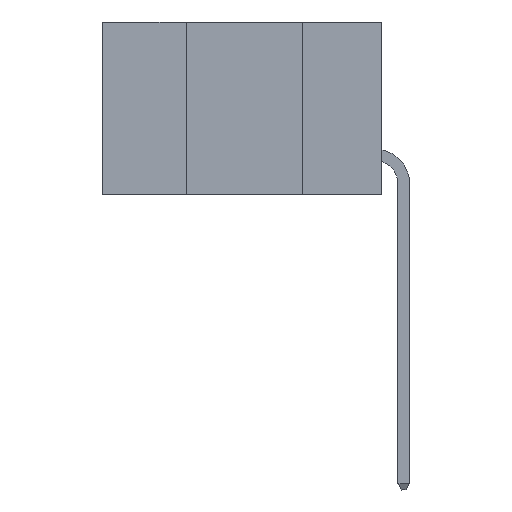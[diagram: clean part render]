
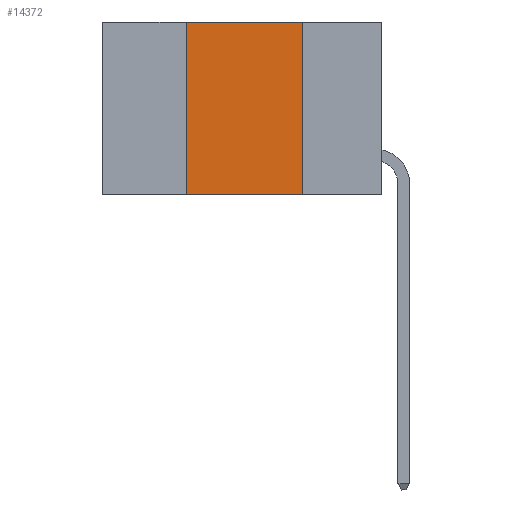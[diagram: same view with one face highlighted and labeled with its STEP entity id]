
A CAD part, left-side view. The second image highlights one B-rep face of the part: STEP entity #14372.
In plain terms, the highlighted planar face has unit normal (-1, 0, 0).
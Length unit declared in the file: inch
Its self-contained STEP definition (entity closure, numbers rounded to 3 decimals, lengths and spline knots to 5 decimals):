
#860 = VECTOR ( 'NONE', #23253, 39.37008 ) ;
#1283 = EDGE_CURVE ( 'NONE', #23550, #6151, #23429, .T. ) ;
#1407 = VERTEX_POINT ( 'NONE', #6427 ) ;
#1477 = LINE ( 'NONE', #4530, #860 ) ;
#1894 = ORIENTED_EDGE ( 'NONE', *, *, #17570, .F. ) ;
#3297 = CARTESIAN_POINT ( 'NONE',  ( 0., 0.42, 0. ) ) ;
#4530 = CARTESIAN_POINT ( 'NONE',  ( 0., 0.17, 0. ) ) ;
#4700 = VECTOR ( 'NONE', #9750, 39.37008 ) ;
#4800 = DIRECTION ( 'NONE',  ( 0., 0., -1. ) ) ;
#6151 = VERTEX_POINT ( 'NONE', #3297 ) ;
#6427 = CARTESIAN_POINT ( 'NONE',  ( 0., 0.17, -0.37 ) ) ;
#7527 = ORIENTED_EDGE ( 'NONE', *, *, #16145, .T. ) ;
#8339 = CARTESIAN_POINT ( 'NONE',  ( 0., 0.6, 0. ) ) ;
#9176 = CARTESIAN_POINT ( 'NONE',  ( 0., 0.17, 0. ) ) ;
#9750 = DIRECTION ( 'NONE',  ( 0., -1., 0. ) ) ;
#11408 = FACE_OUTER_BOUND ( 'NONE', #13101, .T. ) ;
#12465 = CARTESIAN_POINT ( 'NONE',  ( 0., 0.6, 0. ) ) ;
#12761 = AXIS2_PLACEMENT_3D ( 'NONE', #12465, #16162, #4800 ) ;
#13101 = EDGE_LOOP ( 'NONE', ( #18230, #1894, #14459, #7527 ) ) ;
#14244 = LINE ( 'NONE', #22668, #4700 ) ;
#14372 = ADVANCED_FACE ( 'NONE', ( #11408 ), #17868, .F. ) ;
#14459 = ORIENTED_EDGE ( 'NONE', *, *, #1283, .F. ) ;
#14661 = CARTESIAN_POINT ( 'NONE',  ( 0., 0.42, 0. ) ) ;
#15931 = VERTEX_POINT ( 'NONE', #9176 ) ;
#16145 = EDGE_CURVE ( 'NONE', #23550, #1407, #14244, .T. ) ;
#16162 = DIRECTION ( 'NONE',  ( 1., 0., 0. ) ) ;
#17570 = EDGE_CURVE ( 'NONE', #6151, #15931, #18715, .T. ) ;
#17604 = DIRECTION ( 'NONE',  ( 0., -1., 0. ) ) ;
#17868 = PLANE ( 'NONE',  #12761 ) ;
#18230 = ORIENTED_EDGE ( 'NONE', *, *, #23218, .F. ) ;
#18528 = VECTOR ( 'NONE', #22914, 39.37008 ) ;
#18637 = CARTESIAN_POINT ( 'NONE',  ( 0., 0.42, -0.37 ) ) ;
#18715 = LINE ( 'NONE', #8339, #19301 ) ;
#19301 = VECTOR ( 'NONE', #17604, 39.37008 ) ;
#22668 = CARTESIAN_POINT ( 'NONE',  ( 0., 0.6, -0.37 ) ) ;
#22914 = DIRECTION ( 'NONE',  ( 0., 0., 1. ) ) ;
#23218 = EDGE_CURVE ( 'NONE', #15931, #1407, #1477, .T. ) ;
#23253 = DIRECTION ( 'NONE',  ( 0., 0., -1. ) ) ;
#23429 = LINE ( 'NONE', #14661, #18528 ) ;
#23550 = VERTEX_POINT ( 'NONE', #18637 ) ;
